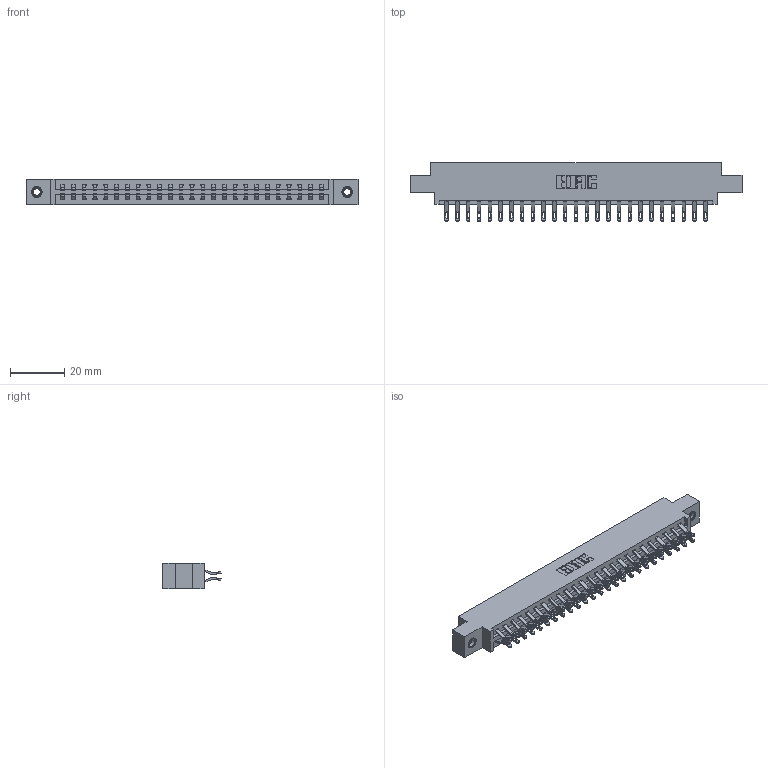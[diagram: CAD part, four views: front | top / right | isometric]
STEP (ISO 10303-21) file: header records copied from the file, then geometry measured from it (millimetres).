
FILE_DESCRIPTION (( 'STEP AP203' ), '1' );
FILE_NAME ('337-050-555-807.STEP', '2018-08-09T21:26:12', ( '' ), ( '' ), 'SwSTEP 2.0', 'SolidWorks 2016', '' );
FILE_SCHEMA (( 'CONFIG_CONTROL_DESIGN' ));
Length unit declared in the file: inch
Products named in the file (4): 337 Part_0.170 Offset - 0.156 Dia-TI; 345-292-001_555 Tail; 345-250-001_345-250-005-103; 337-050-555-807
Assembly tree (53 placements, depth 2):
  337-050-555-807
    337 Part_0.170 Offset - 0.156 Dia-TI
    345-292-001_555 Tail  x50
    345-250-001_345-250-005-103  x2
Bounding box: 122.07 x 21.47 x 9.4 mm (x, y, z)
Volume: 12652.7 mm3; surface area: 14829.1 mm2
Topology: 53 solids, 53 shells, 3178 faces, 9909 edges, 6598 vertices
Faces by surface type: plane 1906, cylinder 1256, cone 12, torus 4
Entity records: 23226 total; most frequent: CARTESIAN_POINT 3943, ORIENTED_EDGE 3842, DIRECTION 3387, EDGE_CURVE 1921, VECTOR 1753, LINE 1753, VERTEX_POINT 1276, AXIS2_PLACEMENT_3D 817
